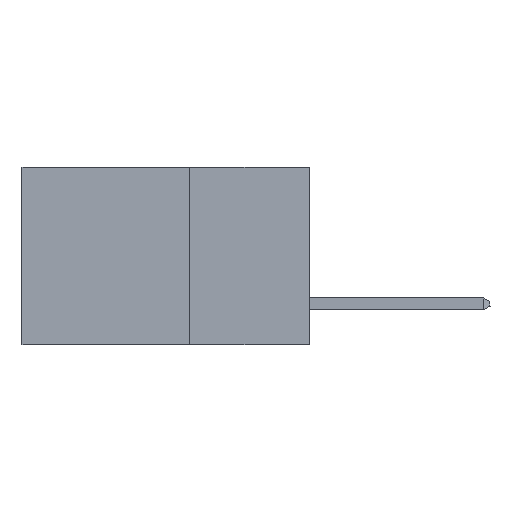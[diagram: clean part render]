
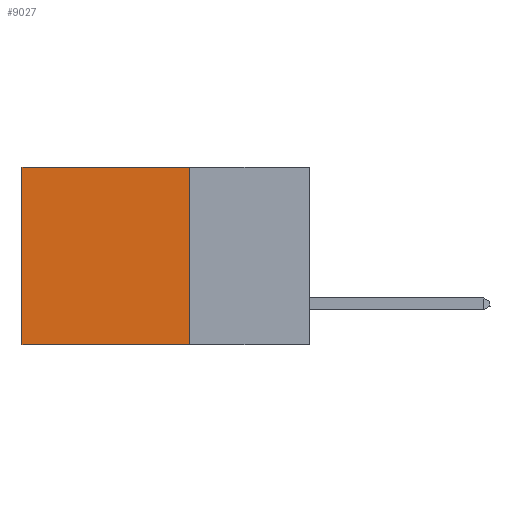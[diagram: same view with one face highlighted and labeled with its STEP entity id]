
A CAD part, left-side view. The second image highlights one B-rep face of the part: STEP entity #9027.
In plain terms, the highlighted planar face has unit normal (-1, 0, 0).
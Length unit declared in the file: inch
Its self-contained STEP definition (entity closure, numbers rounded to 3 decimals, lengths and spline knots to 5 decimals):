
#290 = VERTEX_POINT ( 'NONE', #1534 ) ;
#741 = AXIS2_PLACEMENT_3D ( 'NONE', #9716, #15700, #29947 ) ;
#945 = EDGE_CURVE ( 'NONE', #3571, #11458, #25520, .T. ) ;
#1294 = DIRECTION ( 'NONE',  ( 0., 0., -1. ) ) ;
#1534 = CARTESIAN_POINT ( 'NONE',  ( 0.2875, 0.25, -0.37 ) ) ;
#3571 = VERTEX_POINT ( 'NONE', #36809 ) ;
#5007 = LINE ( 'NONE', #28456, #36094 ) ;
#5259 = CARTESIAN_POINT ( 'NONE',  ( 0.2875, 0.6, 0. ) ) ;
#6586 = ORIENTED_EDGE ( 'NONE', *, *, #32571, .F. ) ;
#7408 = ORIENTED_EDGE ( 'NONE', *, *, #14862, .T. ) ;
#8463 = CARTESIAN_POINT ( 'NONE',  ( 0.2875, 0.25, 0. ) ) ;
#9027 = ADVANCED_FACE ( 'NONE', ( #14399 ), #27070, .F. ) ;
#9716 = CARTESIAN_POINT ( 'NONE',  ( 0.2875, 0.25, 0. ) ) ;
#11445 = DIRECTION ( 'NONE',  ( 0., 0., -1. ) ) ;
#11458 = VERTEX_POINT ( 'NONE', #5259 ) ;
#11856 = CARTESIAN_POINT ( 'NONE',  ( 0.2875, 0.6, -0.37 ) ) ;
#12716 = VECTOR ( 'NONE', #11445, 39.37008 ) ;
#14399 = FACE_OUTER_BOUND ( 'NONE', #38589, .T. ) ;
#14862 = EDGE_CURVE ( 'NONE', #11458, #30022, #36754, .T. ) ;
#15041 = CARTESIAN_POINT ( 'NONE',  ( 0.2875, 0.25, -0.37 ) ) ;
#15700 = DIRECTION ( 'NONE',  ( 1., 0., 0. ) ) ;
#18091 = DIRECTION ( 'NONE',  ( 0., 1., 0. ) ) ;
#21034 = CARTESIAN_POINT ( 'NONE',  ( 0.2875, 0.6, 0. ) ) ;
#23369 = ORIENTED_EDGE ( 'NONE', *, *, #945, .T. ) ;
#25520 = LINE ( 'NONE', #8463, #30207 ) ;
#27070 = PLANE ( 'NONE',  #741 ) ;
#27081 = DIRECTION ( 'NONE',  ( 0., 1., 0. ) ) ;
#27631 = ORIENTED_EDGE ( 'NONE', *, *, #39065, .F. ) ;
#28456 = CARTESIAN_POINT ( 'NONE',  ( 0.2875, 0.25, 0. ) ) ;
#28611 = VECTOR ( 'NONE', #18091, 39.37008 ) ;
#29947 = DIRECTION ( 'NONE',  ( 0., 0., -1. ) ) ;
#30022 = VERTEX_POINT ( 'NONE', #11856 ) ;
#30207 = VECTOR ( 'NONE', #27081, 39.37008 ) ;
#32571 = EDGE_CURVE ( 'NONE', #290, #30022, #32812, .T. ) ;
#32812 = LINE ( 'NONE', #15041, #28611 ) ;
#36094 = VECTOR ( 'NONE', #1294, 39.37008 ) ;
#36754 = LINE ( 'NONE', #21034, #12716 ) ;
#36809 = CARTESIAN_POINT ( 'NONE',  ( 0.2875, 0.25, 0. ) ) ;
#38589 = EDGE_LOOP ( 'NONE', ( #7408, #6586, #27631, #23369 ) ) ;
#39065 = EDGE_CURVE ( 'NONE', #3571, #290, #5007, .T. ) ;
